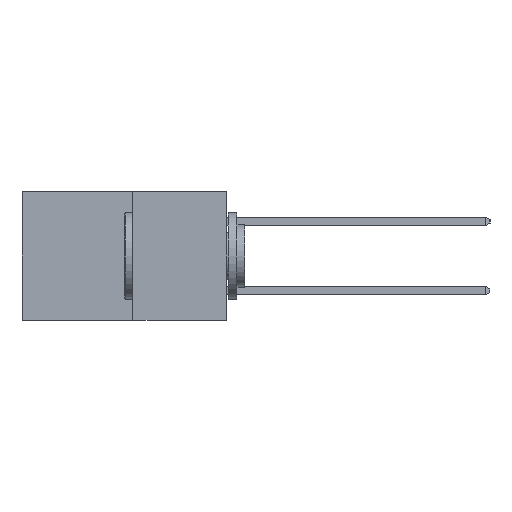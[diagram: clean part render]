
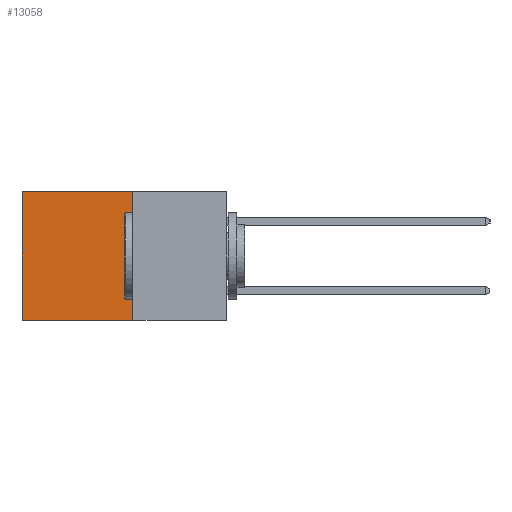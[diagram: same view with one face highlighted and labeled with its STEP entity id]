
A CAD part, left-side view. The second image highlights one B-rep face of the part: STEP entity #13058.
In plain terms, the highlighted planar face has unit normal (-1, 0, 0).
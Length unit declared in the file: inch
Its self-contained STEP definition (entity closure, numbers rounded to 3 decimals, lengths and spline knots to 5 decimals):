
#217 = CARTESIAN_POINT ( 'NONE',  ( 0.277, 0.27, -0.37 ) ) ;
#409 = CARTESIAN_POINT ( 'NONE',  ( 0.277, 0.59, -0.37 ) ) ;
#533 = CARTESIAN_POINT ( 'NONE',  ( 0.277, 0.27, -0.37 ) ) ;
#567 = CARTESIAN_POINT ( 'NONE',  ( 0.277, 0.27, -0.37 ) ) ;
#649 = VERTEX_POINT ( 'NONE', #217 ) ;
#1501 = DIRECTION ( 'NONE',  ( 1., 0., 0. ) ) ;
#1504 = LINE ( 'NONE', #3126, #10032 ) ;
#1543 = LINE ( 'NONE', #567, #1866 ) ;
#1866 = VECTOR ( 'NONE', #9045, 39.37008 ) ;
#2950 = LINE ( 'NONE', #533, #5756 ) ;
#3126 = CARTESIAN_POINT ( 'NONE',  ( 0.277, 0.27, 0. ) ) ;
#3852 = ORIENTED_EDGE ( 'NONE', *, *, #11717, .F. ) ;
#3879 = VERTEX_POINT ( 'NONE', #12901 ) ;
#4093 = EDGE_CURVE ( 'NONE', #3879, #11128, #7423, .T. ) ;
#4188 = ORIENTED_EDGE ( 'NONE', *, *, #10008, .F. ) ;
#4267 = CARTESIAN_POINT ( 'NONE',  ( 0.277, 0.27, 0. ) ) ;
#4629 = FACE_OUTER_BOUND ( 'NONE', #13506, .T. ) ;
#5331 = ORIENTED_EDGE ( 'NONE', *, *, #4093, .T. ) ;
#5756 = VECTOR ( 'NONE', #6840, 39.37008 ) ;
#5920 = VERTEX_POINT ( 'NONE', #4267 ) ;
#5965 = AXIS2_PLACEMENT_3D ( 'NONE', #8914, #1501, #8959 ) ;
#6840 = DIRECTION ( 'NONE',  ( 0., 0., -1. ) ) ;
#7075 = VECTOR ( 'NONE', #8488, 39.37008 ) ;
#7423 = LINE ( 'NONE', #409, #7075 ) ;
#7855 = PLANE ( 'NONE',  #5965 ) ;
#8488 = DIRECTION ( 'NONE',  ( 0., 0., -1. ) ) ;
#8914 = CARTESIAN_POINT ( 'NONE',  ( 0.277, 0.27, -0.37 ) ) ;
#8941 = EDGE_CURVE ( 'NONE', #5920, #3879, #1504, .T. ) ;
#8959 = DIRECTION ( 'NONE',  ( 0., 0., -1. ) ) ;
#9045 = DIRECTION ( 'NONE',  ( 0., 1., 0. ) ) ;
#10008 = EDGE_CURVE ( 'NONE', #5920, #649, #2950, .T. ) ;
#10032 = VECTOR ( 'NONE', #12729, 39.37008 ) ;
#10314 = CARTESIAN_POINT ( 'NONE',  ( 0.277, 0.59, -0.37 ) ) ;
#10572 = ORIENTED_EDGE ( 'NONE', *, *, #8941, .T. ) ;
#11128 = VERTEX_POINT ( 'NONE', #10314 ) ;
#11717 = EDGE_CURVE ( 'NONE', #649, #11128, #1543, .T. ) ;
#12729 = DIRECTION ( 'NONE',  ( 0., 1., 0. ) ) ;
#12901 = CARTESIAN_POINT ( 'NONE',  ( 0.277, 0.59, 0. ) ) ;
#13058 = ADVANCED_FACE ( 'NONE', ( #4629 ), #7855, .F. ) ;
#13506 = EDGE_LOOP ( 'NONE', ( #5331, #3852, #4188, #10572 ) ) ;
